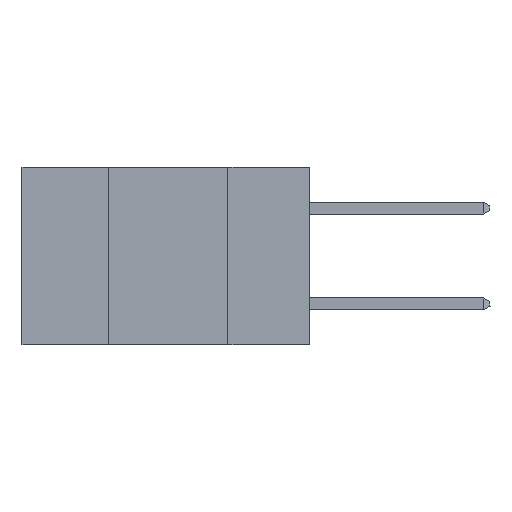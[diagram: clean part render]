
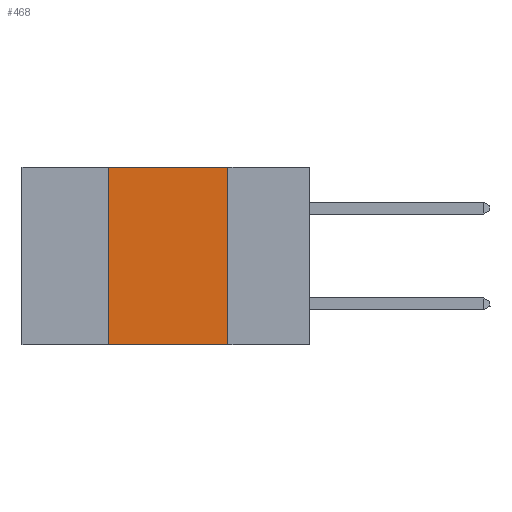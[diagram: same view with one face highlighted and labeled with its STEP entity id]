
A CAD part, left-side view. The second image highlights one B-rep face of the part: STEP entity #468.
In plain terms, the highlighted planar face has unit normal (-1, 0, 0).
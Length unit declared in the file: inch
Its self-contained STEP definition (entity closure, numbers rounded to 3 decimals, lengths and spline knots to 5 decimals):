
#1 = CARTESIAN_POINT ( 'NONE',  ( 0., 0.6, 0. ) ) ;
#468 = ADVANCED_FACE ( 'NONE', ( #3154 ), #4907, .F. ) ;
#681 = VECTOR ( 'NONE', #3849, 39.37008 ) ;
#773 = ORIENTED_EDGE ( 'NONE', *, *, #6748, .T. ) ;
#1377 = CARTESIAN_POINT ( 'NONE',  ( 0., 0.42, 0. ) ) ;
#1382 = VECTOR ( 'NONE', #7200, 39.37008 ) ;
#1453 = VERTEX_POINT ( 'NONE', #8819 ) ;
#1540 = LINE ( 'NONE', #5924, #681 ) ;
#2134 = DIRECTION ( 'NONE',  ( 0., 0., -1. ) ) ;
#2433 = CARTESIAN_POINT ( 'NONE',  ( 0., 0.17, 0. ) ) ;
#2668 = CARTESIAN_POINT ( 'NONE',  ( 0., 0.42, 0. ) ) ;
#3041 = VECTOR ( 'NONE', #3309, 39.37008 ) ;
#3139 = CARTESIAN_POINT ( 'NONE',  ( 0., 0.17, 0. ) ) ;
#3154 = FACE_OUTER_BOUND ( 'NONE', #3394, .T. ) ;
#3155 = VECTOR ( 'NONE', #5577, 39.37008 ) ;
#3309 = DIRECTION ( 'NONE',  ( 0., -1., 0. ) ) ;
#3394 = EDGE_LOOP ( 'NONE', ( #8468, #8197, #4804, #773 ) ) ;
#3849 = DIRECTION ( 'NONE',  ( 0., -1., 0. ) ) ;
#3941 = CARTESIAN_POINT ( 'NONE',  ( 0., 0.42, -0.37 ) ) ;
#4804 = ORIENTED_EDGE ( 'NONE', *, *, #7029, .F. ) ;
#4907 = PLANE ( 'NONE',  #6653 ) ;
#4936 = DIRECTION ( 'NONE',  ( 1., 0., 0. ) ) ;
#5030 = LINE ( 'NONE', #1377, #3155 ) ;
#5217 = EDGE_CURVE ( 'NONE', #6620, #5310, #1540, .T. ) ;
#5310 = VERTEX_POINT ( 'NONE', #3139 ) ;
#5341 = CARTESIAN_POINT ( 'NONE',  ( 0., 0.6, -0.37 ) ) ;
#5374 = VERTEX_POINT ( 'NONE', #3941 ) ;
#5577 = DIRECTION ( 'NONE',  ( 0., 0., 1. ) ) ;
#5886 = LINE ( 'NONE', #5341, #3041 ) ;
#5924 = CARTESIAN_POINT ( 'NONE',  ( 0., 0.6, 0. ) ) ;
#6309 = LINE ( 'NONE', #2433, #1382 ) ;
#6620 = VERTEX_POINT ( 'NONE', #2668 ) ;
#6653 = AXIS2_PLACEMENT_3D ( 'NONE', #1, #4936, #2134 ) ;
#6748 = EDGE_CURVE ( 'NONE', #5374, #1453, #5886, .T. ) ;
#7029 = EDGE_CURVE ( 'NONE', #5374, #6620, #5030, .T. ) ;
#7200 = DIRECTION ( 'NONE',  ( 0., 0., -1. ) ) ;
#8055 = EDGE_CURVE ( 'NONE', #5310, #1453, #6309, .T. ) ;
#8197 = ORIENTED_EDGE ( 'NONE', *, *, #5217, .F. ) ;
#8468 = ORIENTED_EDGE ( 'NONE', *, *, #8055, .F. ) ;
#8819 = CARTESIAN_POINT ( 'NONE',  ( 0., 0.17, -0.37 ) ) ;
